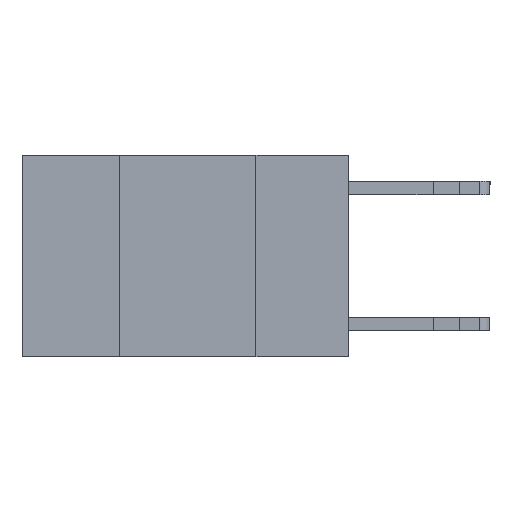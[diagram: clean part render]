
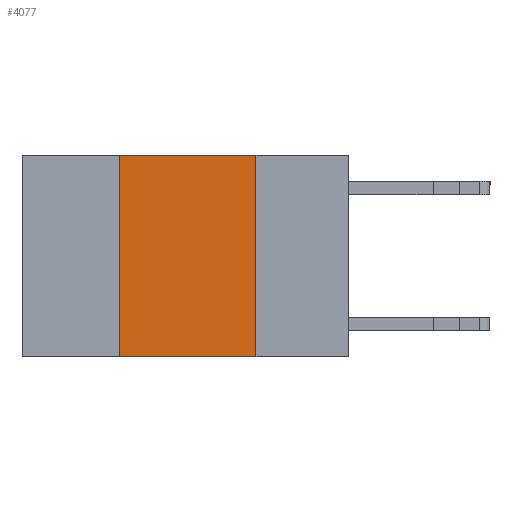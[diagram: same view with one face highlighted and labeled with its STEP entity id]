
A CAD part, left-side view. The second image highlights one B-rep face of the part: STEP entity #4077.
In plain terms, the highlighted planar face has unit normal (-1, 0, 0).
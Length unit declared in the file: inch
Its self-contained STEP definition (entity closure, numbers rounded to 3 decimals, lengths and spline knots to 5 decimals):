
#222 = LINE ( 'NONE', #9278, #5316 ) ;
#800 = ORIENTED_EDGE ( 'NONE', *, *, #12963, .F. ) ;
#1169 = DIRECTION ( 'NONE',  ( 0., 0., 1. ) ) ;
#1214 = CARTESIAN_POINT ( 'NONE',  ( 0., 0.17, -0.37 ) ) ;
#1434 = LINE ( 'NONE', #9344, #10628 ) ;
#1694 = VERTEX_POINT ( 'NONE', #9978 ) ;
#1903 = VERTEX_POINT ( 'NONE', #2578 ) ;
#2127 = PLANE ( 'NONE',  #5273 ) ;
#2578 = CARTESIAN_POINT ( 'NONE',  ( 0., 0.42, -0.37 ) ) ;
#2792 = ORIENTED_EDGE ( 'NONE', *, *, #6421, .F. ) ;
#3217 = DIRECTION ( 'NONE',  ( 0., -1., 0. ) ) ;
#3365 = ORIENTED_EDGE ( 'NONE', *, *, #5429, .F. ) ;
#4077 = ADVANCED_FACE ( 'NONE', ( #8050 ), #2127, .F. ) ;
#5176 = DIRECTION ( 'NONE',  ( 1., 0., 0. ) ) ;
#5245 = CARTESIAN_POINT ( 'NONE',  ( 0., 0.17, 0. ) ) ;
#5273 = AXIS2_PLACEMENT_3D ( 'NONE', #6171, #5176, #11170 ) ;
#5316 = VECTOR ( 'NONE', #3217, 39.37008 ) ;
#5429 = EDGE_CURVE ( 'NONE', #12513, #6964, #5861, .T. ) ;
#5474 = DIRECTION ( 'NONE',  ( 0., -1., 0. ) ) ;
#5861 = LINE ( 'NONE', #5245, #9759 ) ;
#6171 = CARTESIAN_POINT ( 'NONE',  ( 0., 0.6, 0. ) ) ;
#6411 = CARTESIAN_POINT ( 'NONE',  ( 0., 0.42, 0. ) ) ;
#6421 = EDGE_CURVE ( 'NONE', #1694, #12513, #1434, .T. ) ;
#6534 = EDGE_CURVE ( 'NONE', #1903, #6964, #222, .T. ) ;
#6964 = VERTEX_POINT ( 'NONE', #1214 ) ;
#7607 = ORIENTED_EDGE ( 'NONE', *, *, #6534, .T. ) ;
#8050 = FACE_OUTER_BOUND ( 'NONE', #12196, .T. ) ;
#9278 = CARTESIAN_POINT ( 'NONE',  ( 0., 0.6, -0.37 ) ) ;
#9344 = CARTESIAN_POINT ( 'NONE',  ( 0., 0.6, 0. ) ) ;
#9414 = LINE ( 'NONE', #6411, #10143 ) ;
#9759 = VECTOR ( 'NONE', #10990, 39.37008 ) ;
#9978 = CARTESIAN_POINT ( 'NONE',  ( 0., 0.42, 0. ) ) ;
#10143 = VECTOR ( 'NONE', #1169, 39.37008 ) ;
#10628 = VECTOR ( 'NONE', #5474, 39.37008 ) ;
#10990 = DIRECTION ( 'NONE',  ( 0., 0., -1. ) ) ;
#11170 = DIRECTION ( 'NONE',  ( 0., 0., -1. ) ) ;
#12196 = EDGE_LOOP ( 'NONE', ( #3365, #2792, #800, #7607 ) ) ;
#12491 = CARTESIAN_POINT ( 'NONE',  ( 0., 0.17, 0. ) ) ;
#12513 = VERTEX_POINT ( 'NONE', #12491 ) ;
#12963 = EDGE_CURVE ( 'NONE', #1903, #1694, #9414, .T. ) ;
